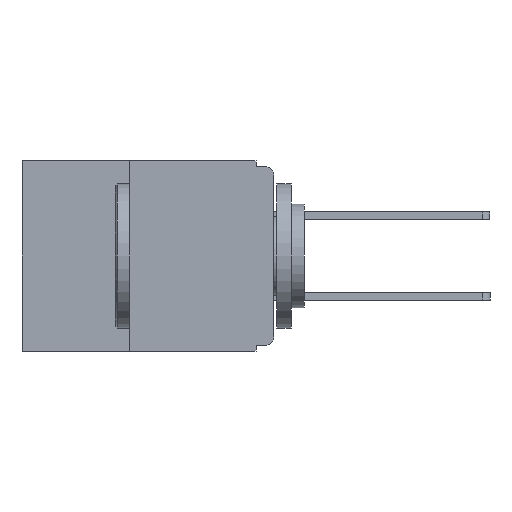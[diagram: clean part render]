
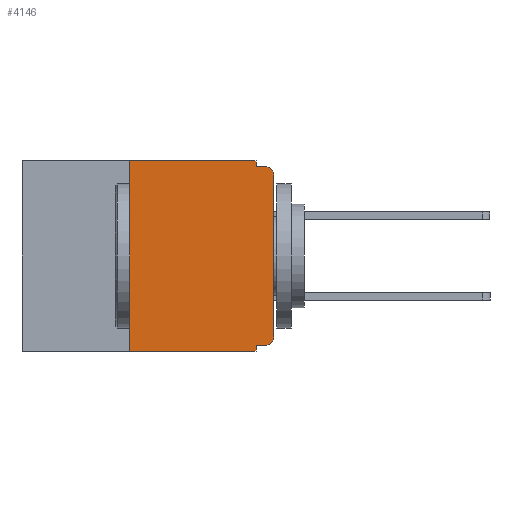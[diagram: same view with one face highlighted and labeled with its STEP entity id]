
A CAD part, left-side view. The second image highlights one B-rep face of the part: STEP entity #4146.
In plain terms, the highlighted planar face has unit normal (-1, 0, 0).
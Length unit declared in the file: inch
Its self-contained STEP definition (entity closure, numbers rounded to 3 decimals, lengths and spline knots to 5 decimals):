
#586 = VECTOR ( 'NONE', #7953, 39.37008 ) ;
#963 = VERTEX_POINT ( 'NONE', #11843 ) ;
#1145 = CARTESIAN_POINT ( 'NONE',  ( 0., 0.437, -0.33 ) ) ;
#1855 = CARTESIAN_POINT ( 'NONE',  ( 0., 0.437, 0. ) ) ;
#1973 = ORIENTED_EDGE ( 'NONE', *, *, #7787, .F. ) ;
#2292 = CARTESIAN_POINT ( 'NONE',  ( 0., 0.015, -0.01 ) ) ;
#2301 = CARTESIAN_POINT ( 'NONE',  ( 0., 0.015, -0.025 ) ) ;
#2534 = AXIS2_PLACEMENT_3D ( 'NONE', #8246, #8245, #8336 ) ;
#2676 = ORIENTED_EDGE ( 'NONE', *, *, #13593, .F. ) ;
#2842 = ORIENTED_EDGE ( 'NONE', *, *, #5042, .T. ) ;
#2898 = VERTEX_POINT ( 'NONE', #2292 ) ;
#2926 = VECTOR ( 'NONE', #10672, 39.37008 ) ;
#2969 = CIRCLE ( 'NONE', #2534, 0.015 ) ;
#3032 = ORIENTED_EDGE ( 'NONE', *, *, #5304, .F. ) ;
#3038 = CARTESIAN_POINT ( 'NONE',  ( 0., 0.25, 0. ) ) ;
#3192 = LINE ( 'NONE', #11732, #6186 ) ;
#3440 = DIRECTION ( 'NONE',  ( 0., 0., -1. ) ) ;
#3600 = CARTESIAN_POINT ( 'NONE',  ( 0., 0.031, -0.33 ) ) ;
#3602 = CARTESIAN_POINT ( 'NONE',  ( 0., 0.25, -0.33 ) ) ;
#3619 = LINE ( 'NONE', #5633, #586 ) ;
#3910 = CARTESIAN_POINT ( 'NONE',  ( 0., 0.437, 0. ) ) ;
#3983 = AXIS2_PLACEMENT_3D ( 'NONE', #2301, #10026, #3440 ) ;
#4109 = EDGE_CURVE ( 'NONE', #5766, #963, #2969, .T. ) ;
#4121 = DIRECTION ( 'NONE',  ( 0., -1., 0. ) ) ;
#4146 = ADVANCED_FACE ( 'NONE', ( #5267 ), #7708, .F. ) ;
#4222 = CARTESIAN_POINT ( 'NONE',  ( 0., 0.031, 0. ) ) ;
#4302 = ORIENTED_EDGE ( 'NONE', *, *, #9614, .F. ) ;
#4683 = VERTEX_POINT ( 'NONE', #6294 ) ;
#5021 = EDGE_LOOP ( 'NONE', ( #2842, #6559, #4302, #10116, #12978, #1973, #13642, #2676, #3032, #11798 ) ) ;
#5042 = EDGE_CURVE ( 'NONE', #963, #4683, #5237, .T. ) ;
#5237 = LINE ( 'NONE', #13360, #13567 ) ;
#5267 = FACE_OUTER_BOUND ( 'NONE', #5021, .T. ) ;
#5304 = EDGE_CURVE ( 'NONE', #5766, #6944, #5940, .T. ) ;
#5444 = LINE ( 'NONE', #3910, #9103 ) ;
#5633 = CARTESIAN_POINT ( 'NONE',  ( 0., 0.25, -0.33 ) ) ;
#5766 = VERTEX_POINT ( 'NONE', #6714 ) ;
#5940 = LINE ( 'NONE', #10734, #2926 ) ;
#6016 = VERTEX_POINT ( 'NONE', #3602 ) ;
#6087 = VERTEX_POINT ( 'NONE', #3038 ) ;
#6186 = VECTOR ( 'NONE', #4121, 39.37008 ) ;
#6294 = CARTESIAN_POINT ( 'NONE',  ( 0., 0., -0.025 ) ) ;
#6309 = AXIS2_PLACEMENT_3D ( 'NONE', #1855, #7663, #7542 ) ;
#6372 = LINE ( 'NONE', #8930, #11772 ) ;
#6559 = ORIENTED_EDGE ( 'NONE', *, *, #7766, .T. ) ;
#6714 = CARTESIAN_POINT ( 'NONE',  ( 0., 0.015, -0.32 ) ) ;
#6797 = DIRECTION ( 'NONE',  ( 0., -1., 0. ) ) ;
#6944 = VERTEX_POINT ( 'NONE', #9514 ) ;
#6955 = VECTOR ( 'NONE', #6797, 39.37008 ) ;
#7376 = DIRECTION ( 'NONE',  ( 0., 0., -1. ) ) ;
#7542 = DIRECTION ( 'NONE',  ( 0., 0., -1. ) ) ;
#7663 = DIRECTION ( 'NONE',  ( 1., 0., 0. ) ) ;
#7708 = PLANE ( 'NONE',  #6309 ) ;
#7766 = EDGE_CURVE ( 'NONE', #4683, #2898, #9813, .T. ) ;
#7787 = EDGE_CURVE ( 'NONE', #6016, #6087, #3619, .T. ) ;
#7869 = VERTEX_POINT ( 'NONE', #3600 ) ;
#7953 = DIRECTION ( 'NONE',  ( 0., 0., 1. ) ) ;
#8107 = LINE ( 'NONE', #12691, #13121 ) ;
#8245 = DIRECTION ( 'NONE',  ( -1., 0., 0. ) ) ;
#8246 = CARTESIAN_POINT ( 'NONE',  ( 0., 0.015, -0.305 ) ) ;
#8336 = DIRECTION ( 'NONE',  ( 0., 0., -1. ) ) ;
#8930 = CARTESIAN_POINT ( 'NONE',  ( 0., 0.031, 0. ) ) ;
#9103 = VECTOR ( 'NONE', #9406, 39.37008 ) ;
#9406 = DIRECTION ( 'NONE',  ( 0., -1., 0. ) ) ;
#9514 = CARTESIAN_POINT ( 'NONE',  ( 0., 0.031, -0.32 ) ) ;
#9614 = EDGE_CURVE ( 'NONE', #11673, #2898, #3192, .T. ) ;
#9675 = VERTEX_POINT ( 'NONE', #4222 ) ;
#9813 = CIRCLE ( 'NONE', #3983, 0.015 ) ;
#9966 = DIRECTION ( 'NONE',  ( 0., 0., -1. ) ) ;
#10026 = DIRECTION ( 'NONE',  ( -1., 0., 0. ) ) ;
#10079 = EDGE_CURVE ( 'NONE', #6087, #9675, #5444, .T. ) ;
#10116 = ORIENTED_EDGE ( 'NONE', *, *, #13243, .F. ) ;
#10672 = DIRECTION ( 'NONE',  ( 0., 1., 0. ) ) ;
#10734 = CARTESIAN_POINT ( 'NONE',  ( 0., 0., -0.32 ) ) ;
#11198 = CARTESIAN_POINT ( 'NONE',  ( 0., 0.031, -0.01 ) ) ;
#11594 = EDGE_CURVE ( 'NONE', #6016, #7869, #13014, .T. ) ;
#11673 = VERTEX_POINT ( 'NONE', #11198 ) ;
#11732 = CARTESIAN_POINT ( 'NONE',  ( 0., 0., -0.01 ) ) ;
#11772 = VECTOR ( 'NONE', #9966, 39.37008 ) ;
#11798 = ORIENTED_EDGE ( 'NONE', *, *, #4109, .T. ) ;
#11843 = CARTESIAN_POINT ( 'NONE',  ( 0., 0., -0.305 ) ) ;
#12691 = CARTESIAN_POINT ( 'NONE',  ( 0., 0.031, -0.33 ) ) ;
#12978 = ORIENTED_EDGE ( 'NONE', *, *, #10079, .F. ) ;
#13014 = LINE ( 'NONE', #1145, #6955 ) ;
#13121 = VECTOR ( 'NONE', #7376, 39.37008 ) ;
#13243 = EDGE_CURVE ( 'NONE', #9675, #11673, #6372, .T. ) ;
#13267 = DIRECTION ( 'NONE',  ( 0., 0., 1. ) ) ;
#13360 = CARTESIAN_POINT ( 'NONE',  ( 0., 0., 0. ) ) ;
#13567 = VECTOR ( 'NONE', #13267, 39.37008 ) ;
#13593 = EDGE_CURVE ( 'NONE', #6944, #7869, #8107, .T. ) ;
#13642 = ORIENTED_EDGE ( 'NONE', *, *, #11594, .T. ) ;
